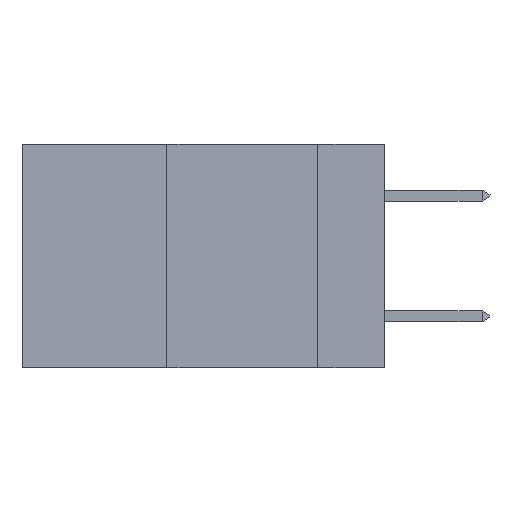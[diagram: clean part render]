
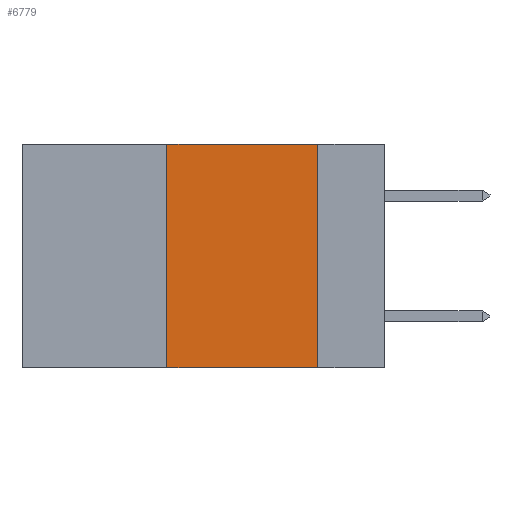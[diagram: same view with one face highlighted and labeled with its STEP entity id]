
A CAD part, left-side view. The second image highlights one B-rep face of the part: STEP entity #6779.
In plain terms, the highlighted planar face has unit normal (-1, 0, 0).
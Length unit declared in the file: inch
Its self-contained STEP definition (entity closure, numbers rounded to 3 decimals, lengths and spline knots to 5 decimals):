
#803 = ORIENTED_EDGE ( 'NONE', *, *, #17715, .F. ) ;
#1038 = VECTOR ( 'NONE', #11310, 39.37008 ) ;
#1045 = PLANE ( 'NONE',  #2080 ) ;
#1715 = CARTESIAN_POINT ( 'NONE',  ( 0., 0.36, 0. ) ) ;
#2080 = AXIS2_PLACEMENT_3D ( 'NONE', #12732, #14404, #11222 ) ;
#3191 = VERTEX_POINT ( 'NONE', #4134 ) ;
#3531 = LINE ( 'NONE', #19075, #18335 ) ;
#3865 = FACE_OUTER_BOUND ( 'NONE', #16292, .T. ) ;
#4134 = CARTESIAN_POINT ( 'NONE',  ( 0., 0.11, -0.37 ) ) ;
#4707 = LINE ( 'NONE', #8840, #18202 ) ;
#5286 = VERTEX_POINT ( 'NONE', #16821 ) ;
#6423 = EDGE_CURVE ( 'NONE', #5286, #13922, #13801, .T. ) ;
#6779 = ADVANCED_FACE ( 'NONE', ( #3865 ), #1045, .F. ) ;
#6965 = ORIENTED_EDGE ( 'NONE', *, *, #6423, .F. ) ;
#8572 = ORIENTED_EDGE ( 'NONE', *, *, #13696, .T. ) ;
#8840 = CARTESIAN_POINT ( 'NONE',  ( 0., 0.6, 0. ) ) ;
#8865 = VECTOR ( 'NONE', #15005, 39.37008 ) ;
#9197 = DIRECTION ( 'NONE',  ( 0., 0., -1. ) ) ;
#10564 = CARTESIAN_POINT ( 'NONE',  ( 0., 0.11, 0. ) ) ;
#11222 = DIRECTION ( 'NONE',  ( 0., 0., -1. ) ) ;
#11310 = DIRECTION ( 'NONE',  ( 0., -1., 0. ) ) ;
#12682 = VERTEX_POINT ( 'NONE', #10564 ) ;
#12732 = CARTESIAN_POINT ( 'NONE',  ( 0., 0.6, 0. ) ) ;
#13696 = EDGE_CURVE ( 'NONE', #5286, #3191, #14295, .T. ) ;
#13801 = LINE ( 'NONE', #1715, #8865 ) ;
#13922 = VERTEX_POINT ( 'NONE', #20306 ) ;
#14295 = LINE ( 'NONE', #16183, #1038 ) ;
#14404 = DIRECTION ( 'NONE',  ( 1., 0., 0. ) ) ;
#15005 = DIRECTION ( 'NONE',  ( 0., 0., 1. ) ) ;
#15387 = DIRECTION ( 'NONE',  ( 0., -1., 0. ) ) ;
#16183 = CARTESIAN_POINT ( 'NONE',  ( 0., 0.6, -0.37 ) ) ;
#16292 = EDGE_LOOP ( 'NONE', ( #803, #18249, #6965, #8572 ) ) ;
#16821 = CARTESIAN_POINT ( 'NONE',  ( 0., 0.36, -0.37 ) ) ;
#17715 = EDGE_CURVE ( 'NONE', #12682, #3191, #3531, .T. ) ;
#18202 = VECTOR ( 'NONE', #15387, 39.37008 ) ;
#18249 = ORIENTED_EDGE ( 'NONE', *, *, #20409, .F. ) ;
#18335 = VECTOR ( 'NONE', #9197, 39.37008 ) ;
#19075 = CARTESIAN_POINT ( 'NONE',  ( 0., 0.11, 0. ) ) ;
#20306 = CARTESIAN_POINT ( 'NONE',  ( 0., 0.36, 0. ) ) ;
#20409 = EDGE_CURVE ( 'NONE', #13922, #12682, #4707, .T. ) ;
